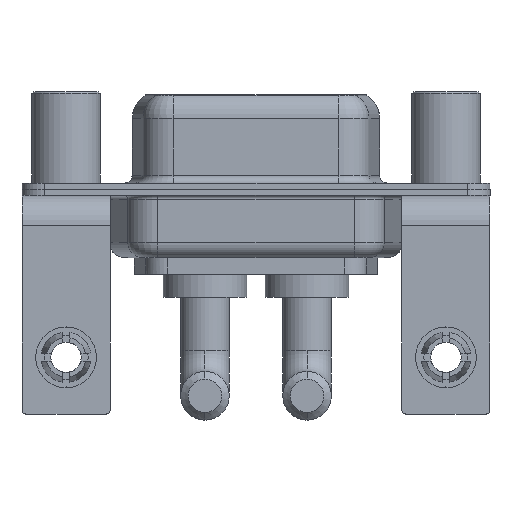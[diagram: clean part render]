
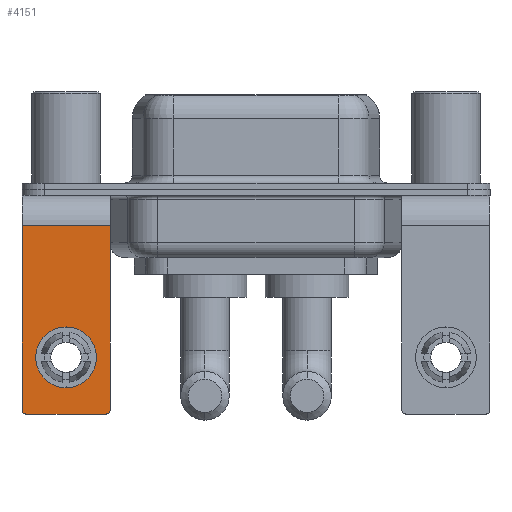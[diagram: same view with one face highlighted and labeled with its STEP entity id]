
A CAD part, front view. The second image highlights one B-rep face of the part: STEP entity #4151.
In plain terms, the highlighted planar face has unit normal (0, -1, 0).
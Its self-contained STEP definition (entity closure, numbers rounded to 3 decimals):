
#189 = DIRECTION ( 'NONE',  ( 0., 1., 0. ) ) ;
#372 = CARTESIAN_POINT ( 'NONE',  ( -2.65, -6.25, -14.55 ) ) ;
#807 = ORIENTED_EDGE ( 'NONE', *, *, #10399, .T. ) ;
#974 = VERTEX_POINT ( 'NONE', #8788 ) ;
#1163 = ORIENTED_EDGE ( 'NONE', *, *, #2037, .T. ) ;
#1209 = EDGE_CURVE ( 'NONE', #15676, #12730, #1861, .T. ) ;
#1211 = VERTEX_POINT ( 'NONE', #14483 ) ;
#1263 = FACE_OUTER_BOUND ( 'NONE', #11331, .T. ) ;
#1483 = CIRCLE ( 'NONE', #13599, 2. ) ;
#1806 = CIRCLE ( 'NONE', #8901, 0.25 ) ;
#1861 = LINE ( 'NONE', #9473, #2790 ) ;
#2037 = EDGE_CURVE ( 'NONE', #9599, #7418, #9036, .T. ) ;
#2039 = CARTESIAN_POINT ( 'NONE',  ( 2.9, -6.25, -2.4 ) ) ;
#2500 = LINE ( 'NONE', #8589, #9702 ) ;
#2790 = VECTOR ( 'NONE', #12995, 1000. ) ;
#2907 = FACE_BOUND ( 'NONE', #14807, .T. ) ;
#3183 = ORIENTED_EDGE ( 'NONE', *, *, #11395, .F. ) ;
#3582 = VERTEX_POINT ( 'NONE', #16061 ) ;
#3954 = DIRECTION ( 'NONE',  ( 0., 0., 1. ) ) ;
#4007 = DIRECTION ( 'NONE',  ( 0., 0., 1. ) ) ;
#4151 = ADVANCED_FACE ( 'NONE', ( #2907, #1263 ), #7601, .F. ) ;
#4339 = CARTESIAN_POINT ( 'NONE',  ( 0., -6.25, -11.07 ) ) ;
#5027 = VERTEX_POINT ( 'NONE', #6250 ) ;
#5099 = ORIENTED_EDGE ( 'NONE', *, *, #1209, .T. ) ;
#5830 = DIRECTION ( 'NONE',  ( 0., 0., -1. ) ) ;
#5907 = ORIENTED_EDGE ( 'NONE', *, *, #15253, .T. ) ;
#6250 = CARTESIAN_POINT ( 'NONE',  ( -2.65, -6.25, -14.8 ) ) ;
#6388 = AXIS2_PLACEMENT_3D ( 'NONE', #4339, #10647, #4007 ) ;
#6800 = DIRECTION ( 'NONE',  ( 0., -1., 0. ) ) ;
#6997 = CARTESIAN_POINT ( 'NONE',  ( 2.9, -6.25, -2.4 ) ) ;
#7151 = LINE ( 'NONE', #6997, #10214 ) ;
#7418 = VERTEX_POINT ( 'NONE', #12383 ) ;
#7494 = DIRECTION ( 'NONE',  ( 0., 1., 0. ) ) ;
#7601 = PLANE ( 'NONE',  #12665 ) ;
#7832 = ORIENTED_EDGE ( 'NONE', *, *, #9991, .T. ) ;
#8337 = EDGE_CURVE ( 'NONE', #974, #15676, #9641, .T. ) ;
#8538 = DIRECTION ( 'NONE',  ( -1., 0., 0. ) ) ;
#8589 = CARTESIAN_POINT ( 'NONE',  ( 2.9, -6.25, -14.8 ) ) ;
#8788 = CARTESIAN_POINT ( 'NONE',  ( 2.9, -6.25, -2.4 ) ) ;
#8843 = DIRECTION ( 'NONE',  ( -1., 0., 0. ) ) ;
#8901 = AXIS2_PLACEMENT_3D ( 'NONE', #372, #6800, #13964 ) ;
#9036 = CIRCLE ( 'NONE', #6388, 2. ) ;
#9473 = CARTESIAN_POINT ( 'NONE',  ( -2.9, -6.25, -2.4 ) ) ;
#9594 = CARTESIAN_POINT ( 'NONE',  ( -2.9, -6.25, -14.55 ) ) ;
#9599 = VERTEX_POINT ( 'NONE', #13062 ) ;
#9641 = LINE ( 'NONE', #2039, #12424 ) ;
#9702 = VECTOR ( 'NONE', #8843, 1000. ) ;
#9991 = EDGE_CURVE ( 'NONE', #3582, #1211, #14303, .T. ) ;
#9997 = DIRECTION ( 'NONE',  ( 0., 0., 1. ) ) ;
#10214 = VECTOR ( 'NONE', #5830, 1000. ) ;
#10376 = AXIS2_PLACEMENT_3D ( 'NONE', #14862, #15189, #3954 ) ;
#10399 = EDGE_CURVE ( 'NONE', #7418, #9599, #1483, .T. ) ;
#10647 = DIRECTION ( 'NONE',  ( 0., 1., 0. ) ) ;
#10672 = ORIENTED_EDGE ( 'NONE', *, *, #8337, .T. ) ;
#11152 = CARTESIAN_POINT ( 'NONE',  ( 0., -6.25, -11.07 ) ) ;
#11331 = EDGE_LOOP ( 'NONE', ( #5099, #5907, #3183, #7832, #13500, #10672 ) ) ;
#11395 = EDGE_CURVE ( 'NONE', #3582, #5027, #2500, .T. ) ;
#12383 = CARTESIAN_POINT ( 'NONE',  ( 0., -6.25, -13.07 ) ) ;
#12424 = VECTOR ( 'NONE', #8538, 1000. ) ;
#12640 = DIRECTION ( 'NONE',  ( 0., 0., 1. ) ) ;
#12665 = AXIS2_PLACEMENT_3D ( 'NONE', #14045, #189, #12640 ) ;
#12730 = VERTEX_POINT ( 'NONE', #9594 ) ;
#12995 = DIRECTION ( 'NONE',  ( 0., 0., -1. ) ) ;
#13062 = CARTESIAN_POINT ( 'NONE',  ( 0., -6.25, -9.07 ) ) ;
#13141 = EDGE_CURVE ( 'NONE', #974, #1211, #7151, .T. ) ;
#13500 = ORIENTED_EDGE ( 'NONE', *, *, #13141, .F. ) ;
#13599 = AXIS2_PLACEMENT_3D ( 'NONE', #11152, #7494, #9997 ) ;
#13964 = DIRECTION ( 'NONE',  ( 0., 0., 1. ) ) ;
#14045 = CARTESIAN_POINT ( 'NONE',  ( 2.9, -6.25, -2.4 ) ) ;
#14283 = CARTESIAN_POINT ( 'NONE',  ( -2.9, -6.25, -2.4 ) ) ;
#14303 = CIRCLE ( 'NONE', #10376, 0.25 ) ;
#14483 = CARTESIAN_POINT ( 'NONE',  ( 2.9, -6.25, -14.55 ) ) ;
#14807 = EDGE_LOOP ( 'NONE', ( #807, #1163 ) ) ;
#14862 = CARTESIAN_POINT ( 'NONE',  ( 2.65, -6.25, -14.55 ) ) ;
#15189 = DIRECTION ( 'NONE',  ( 0., -1., 0. ) ) ;
#15253 = EDGE_CURVE ( 'NONE', #12730, #5027, #1806, .T. ) ;
#15676 = VERTEX_POINT ( 'NONE', #14283 ) ;
#16061 = CARTESIAN_POINT ( 'NONE',  ( 2.65, -6.25, -14.8 ) ) ;
